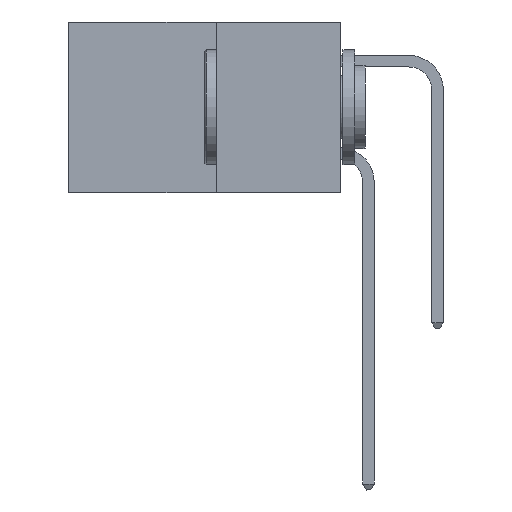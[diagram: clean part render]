
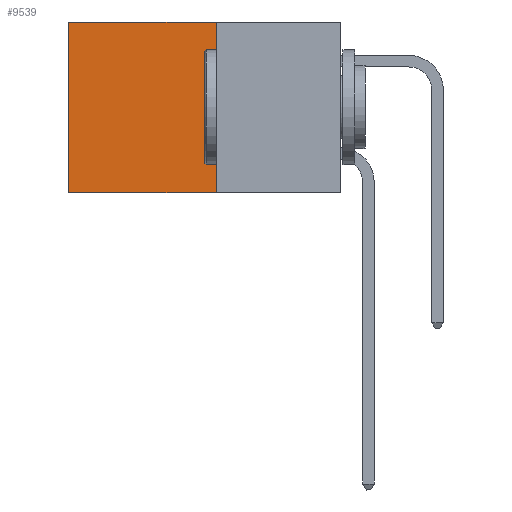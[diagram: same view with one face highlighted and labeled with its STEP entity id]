
A CAD part, left-side view. The second image highlights one B-rep face of the part: STEP entity #9539.
In plain terms, the highlighted planar face has unit normal (-1, 0, 0).
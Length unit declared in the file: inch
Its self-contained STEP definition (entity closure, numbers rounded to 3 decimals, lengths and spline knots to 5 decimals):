
#155 = LINE ( 'NONE', #8361, #8373 ) ;
#1459 = CARTESIAN_POINT ( 'NONE',  ( 0.277, 0.27, -0.37 ) ) ;
#3471 = VERTEX_POINT ( 'NONE', #1459 ) ;
#4607 = CARTESIAN_POINT ( 'NONE',  ( 0.277, 0.59, -0.37 ) ) ;
#4833 = ORIENTED_EDGE ( 'NONE', *, *, #21374, .F. ) ;
#6144 = ORIENTED_EDGE ( 'NONE', *, *, #14672, .F. ) ;
#6980 = DIRECTION ( 'NONE',  ( 0., 0., -1. ) ) ;
#7905 = LINE ( 'NONE', #10334, #16508 ) ;
#8361 = CARTESIAN_POINT ( 'NONE',  ( 0.277, 0.27, -0.37 ) ) ;
#8373 = VECTOR ( 'NONE', #10099, 39.37008 ) ;
#8428 = EDGE_LOOP ( 'NONE', ( #21857, #4833, #6144, #13834 ) ) ;
#9539 = ADVANCED_FACE ( 'NONE', ( #9583 ), #14352, .F. ) ;
#9583 = FACE_OUTER_BOUND ( 'NONE', #8428, .T. ) ;
#10038 = AXIS2_PLACEMENT_3D ( 'NONE', #14420, #14054, #13972 ) ;
#10099 = DIRECTION ( 'NONE',  ( 0., 1., 0. ) ) ;
#10334 = CARTESIAN_POINT ( 'NONE',  ( 0.277, 0.27, 0. ) ) ;
#11157 = CARTESIAN_POINT ( 'NONE',  ( 0.277, 0.59, 0. ) ) ;
#11788 = VECTOR ( 'NONE', #6980, 39.37008 ) ;
#12064 = DIRECTION ( 'NONE',  ( 0., 1., 0. ) ) ;
#12836 = DIRECTION ( 'NONE',  ( 0., 0., -1. ) ) ;
#13460 = VERTEX_POINT ( 'NONE', #17727 ) ;
#13834 = ORIENTED_EDGE ( 'NONE', *, *, #21467, .T. ) ;
#13972 = DIRECTION ( 'NONE',  ( 0., 0., -1. ) ) ;
#14054 = DIRECTION ( 'NONE',  ( 1., 0., 0. ) ) ;
#14352 = PLANE ( 'NONE',  #10038 ) ;
#14420 = CARTESIAN_POINT ( 'NONE',  ( 0.277, 0.27, -0.37 ) ) ;
#14672 = EDGE_CURVE ( 'NONE', #13460, #3471, #15768, .T. ) ;
#15639 = EDGE_CURVE ( 'NONE', #19959, #20124, #17427, .T. ) ;
#15768 = LINE ( 'NONE', #17319, #11788 ) ;
#16508 = VECTOR ( 'NONE', #12064, 39.37008 ) ;
#17319 = CARTESIAN_POINT ( 'NONE',  ( 0.277, 0.27, -0.37 ) ) ;
#17427 = LINE ( 'NONE', #19548, #20297 ) ;
#17727 = CARTESIAN_POINT ( 'NONE',  ( 0.277, 0.27, 0. ) ) ;
#19548 = CARTESIAN_POINT ( 'NONE',  ( 0.277, 0.59, -0.37 ) ) ;
#19959 = VERTEX_POINT ( 'NONE', #11157 ) ;
#20124 = VERTEX_POINT ( 'NONE', #4607 ) ;
#20297 = VECTOR ( 'NONE', #12836, 39.37008 ) ;
#21374 = EDGE_CURVE ( 'NONE', #3471, #20124, #155, .T. ) ;
#21467 = EDGE_CURVE ( 'NONE', #13460, #19959, #7905, .T. ) ;
#21857 = ORIENTED_EDGE ( 'NONE', *, *, #15639, .T. ) ;
